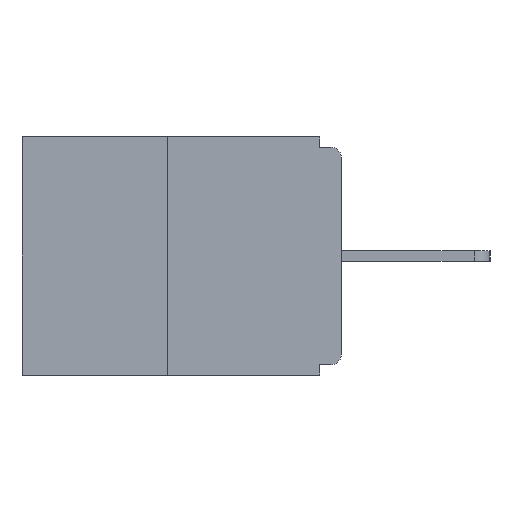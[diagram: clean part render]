
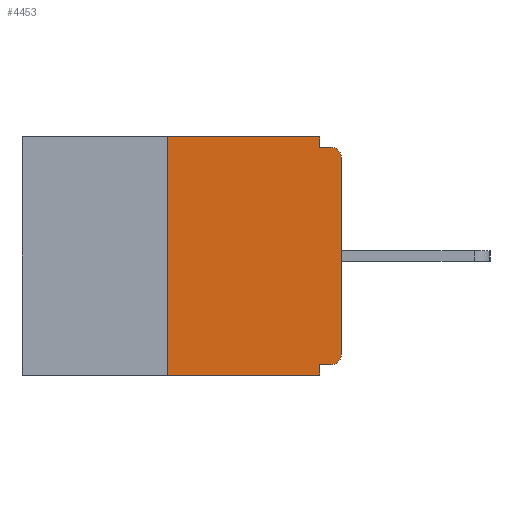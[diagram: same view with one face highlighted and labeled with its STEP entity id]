
A CAD part, left-side view. The second image highlights one B-rep face of the part: STEP entity #4453.
In plain terms, the highlighted planar face has unit normal (-1, 0, 0).
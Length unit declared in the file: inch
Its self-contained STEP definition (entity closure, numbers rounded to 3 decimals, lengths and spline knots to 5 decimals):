
#8 = LINE ( 'NONE', #10713, #6682 ) ;
#269 = DIRECTION ( 'NONE',  ( 0., 1., 0. ) ) ;
#326 = DIRECTION ( 'NONE',  ( 0., 0., 1. ) ) ;
#384 = CARTESIAN_POINT ( 'NONE',  ( 0., 0.031, 0. ) ) ;
#438 = CARTESIAN_POINT ( 'NONE',  ( 0., 0., 0. ) ) ;
#724 = VERTEX_POINT ( 'NONE', #5365 ) ;
#975 = VERTEX_POINT ( 'NONE', #5776 ) ;
#1063 = CARTESIAN_POINT ( 'NONE',  ( 0., 0.46, 0. ) ) ;
#1149 = DIRECTION ( 'NONE',  ( 1., 0., 0. ) ) ;
#1249 = VECTOR ( 'NONE', #2145, 39.37008 ) ;
#1278 = CARTESIAN_POINT ( 'NONE',  ( 0., 0., -0.03 ) ) ;
#1339 = VERTEX_POINT ( 'NONE', #5195 ) ;
#1368 = EDGE_CURVE ( 'NONE', #9787, #1339, #12367, .T. ) ;
#1456 = ORIENTED_EDGE ( 'NONE', *, *, #8179, .F. ) ;
#1618 = EDGE_LOOP ( 'NONE', ( #14758, #1456, #8422, #11804, #8823, #12191, #9235, #12579, #12971, #16280 ) ) ;
#1750 = DIRECTION ( 'NONE',  ( 0., 0., -1. ) ) ;
#1788 = EDGE_CURVE ( 'NONE', #2261, #724, #4087, .T. ) ;
#2145 = DIRECTION ( 'NONE',  ( 0., 0., -1. ) ) ;
#2261 = VERTEX_POINT ( 'NONE', #15554 ) ;
#2267 = VECTOR ( 'NONE', #269, 39.37008 ) ;
#3243 = VERTEX_POINT ( 'NONE', #8943 ) ;
#3604 = EDGE_CURVE ( 'NONE', #15997, #6778, #8, .T. ) ;
#3936 = EDGE_CURVE ( 'NONE', #975, #6778, #5232, .T. ) ;
#3998 = DIRECTION ( 'NONE',  ( 0., -1., 0. ) ) ;
#4087 = LINE ( 'NONE', #7859, #10509 ) ;
#4453 = ADVANCED_FACE ( 'NONE', ( #13382 ), #13255, .F. ) ;
#4956 = CARTESIAN_POINT ( 'NONE',  ( 0., 0.46, 0. ) ) ;
#5195 = CARTESIAN_POINT ( 'NONE',  ( 0., 0.031, 0. ) ) ;
#5232 = LINE ( 'NONE', #16625, #1249 ) ;
#5263 = DIRECTION ( 'NONE',  ( -1., 0., 0. ) ) ;
#5365 = CARTESIAN_POINT ( 'NONE',  ( 0., 0.015, -0.015 ) ) ;
#5463 = EDGE_CURVE ( 'NONE', #3243, #975, #15109, .T. ) ;
#5743 = LINE ( 'NONE', #12473, #15814 ) ;
#5776 = CARTESIAN_POINT ( 'NONE',  ( 0., 0.031, -0.328 ) ) ;
#6431 = DIRECTION ( 'NONE',  ( 0., 0., -1. ) ) ;
#6453 = DIRECTION ( 'NONE',  ( -1., 0., 0. ) ) ;
#6478 = CIRCLE ( 'NONE', #13211, 0.015 ) ;
#6487 = CARTESIAN_POINT ( 'NONE',  ( 0., 0.015, -0.313 ) ) ;
#6682 = VECTOR ( 'NONE', #7231, 39.37008 ) ;
#6778 = VERTEX_POINT ( 'NONE', #11249 ) ;
#6807 = AXIS2_PLACEMENT_3D ( 'NONE', #1063, #1149, #12479 ) ;
#7064 = CIRCLE ( 'NONE', #8870, 0.015 ) ;
#7231 = DIRECTION ( 'NONE',  ( 0., -1., 0. ) ) ;
#7859 = CARTESIAN_POINT ( 'NONE',  ( 0., 0., -0.015 ) ) ;
#7917 = VERTEX_POINT ( 'NONE', #15871 ) ;
#8179 = EDGE_CURVE ( 'NONE', #15997, #9787, #5743, .T. ) ;
#8422 = ORIENTED_EDGE ( 'NONE', *, *, #3604, .T. ) ;
#8494 = DIRECTION ( 'NONE',  ( 0., -1., 0. ) ) ;
#8823 = ORIENTED_EDGE ( 'NONE', *, *, #5463, .F. ) ;
#8870 = AXIS2_PLACEMENT_3D ( 'NONE', #12866, #5263, #14158 ) ;
#8943 = CARTESIAN_POINT ( 'NONE',  ( 0., 0.015, -0.328 ) ) ;
#9007 = VECTOR ( 'NONE', #3998, 39.37008 ) ;
#9181 = CARTESIAN_POINT ( 'NONE',  ( 0., 0., -0.328 ) ) ;
#9235 = ORIENTED_EDGE ( 'NONE', *, *, #10476, .T. ) ;
#9787 = VERTEX_POINT ( 'NONE', #11869 ) ;
#10130 = EDGE_CURVE ( 'NONE', #3243, #7917, #6478, .T. ) ;
#10476 = EDGE_CURVE ( 'NONE', #7917, #14646, #14769, .T. ) ;
#10509 = VECTOR ( 'NONE', #8494, 39.37008 ) ;
#10618 = VECTOR ( 'NONE', #326, 39.37008 ) ;
#10713 = CARTESIAN_POINT ( 'NONE',  ( 0., 0.46, -0.343 ) ) ;
#10719 = EDGE_CURVE ( 'NONE', #14646, #724, #7064, .T. ) ;
#11249 = CARTESIAN_POINT ( 'NONE',  ( 0., 0.031, -0.343 ) ) ;
#11428 = EDGE_CURVE ( 'NONE', #1339, #2261, #13558, .T. ) ;
#11804 = ORIENTED_EDGE ( 'NONE', *, *, #3936, .F. ) ;
#11869 = CARTESIAN_POINT ( 'NONE',  ( 0., 0.25, 0. ) ) ;
#12191 = ORIENTED_EDGE ( 'NONE', *, *, #10130, .T. ) ;
#12287 = DIRECTION ( 'NONE',  ( 0., 0., 1. ) ) ;
#12367 = LINE ( 'NONE', #4956, #9007 ) ;
#12473 = CARTESIAN_POINT ( 'NONE',  ( 0., 0.25, 0. ) ) ;
#12479 = DIRECTION ( 'NONE',  ( 0., 0., -1. ) ) ;
#12579 = ORIENTED_EDGE ( 'NONE', *, *, #10719, .T. ) ;
#12866 = CARTESIAN_POINT ( 'NONE',  ( 0., 0.015, -0.03 ) ) ;
#12971 = ORIENTED_EDGE ( 'NONE', *, *, #1788, .F. ) ;
#13211 = AXIS2_PLACEMENT_3D ( 'NONE', #6487, #6453, #6431 ) ;
#13255 = PLANE ( 'NONE',  #6807 ) ;
#13382 = FACE_OUTER_BOUND ( 'NONE', #1618, .T. ) ;
#13558 = LINE ( 'NONE', #384, #16432 ) ;
#14158 = DIRECTION ( 'NONE',  ( 0., 0., -1. ) ) ;
#14352 = CARTESIAN_POINT ( 'NONE',  ( 0., 0.25, -0.343 ) ) ;
#14646 = VERTEX_POINT ( 'NONE', #1278 ) ;
#14758 = ORIENTED_EDGE ( 'NONE', *, *, #1368, .F. ) ;
#14769 = LINE ( 'NONE', #438, #10618 ) ;
#15109 = LINE ( 'NONE', #9181, #2267 ) ;
#15554 = CARTESIAN_POINT ( 'NONE',  ( 0., 0.031, -0.015 ) ) ;
#15814 = VECTOR ( 'NONE', #12287, 39.37008 ) ;
#15871 = CARTESIAN_POINT ( 'NONE',  ( 0., 0., -0.313 ) ) ;
#15997 = VERTEX_POINT ( 'NONE', #14352 ) ;
#16280 = ORIENTED_EDGE ( 'NONE', *, *, #11428, .F. ) ;
#16432 = VECTOR ( 'NONE', #1750, 39.37008 ) ;
#16625 = CARTESIAN_POINT ( 'NONE',  ( 0., 0.031, -0.343 ) ) ;
